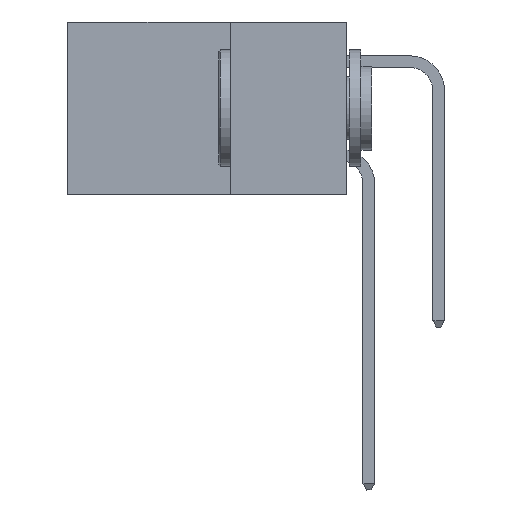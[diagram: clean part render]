
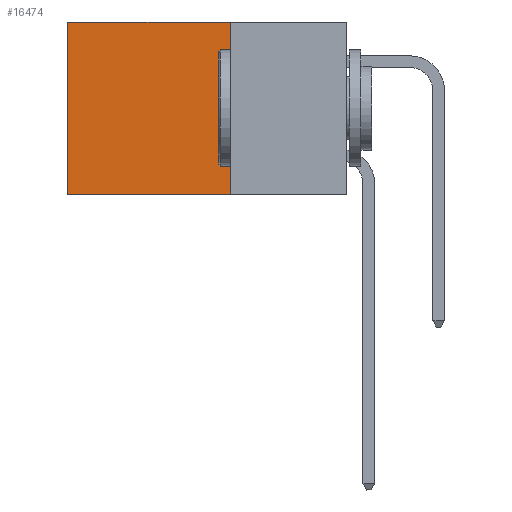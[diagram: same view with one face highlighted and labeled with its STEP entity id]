
A CAD part, left-side view. The second image highlights one B-rep face of the part: STEP entity #16474.
In plain terms, the highlighted planar face has unit normal (-1, 0, 0).
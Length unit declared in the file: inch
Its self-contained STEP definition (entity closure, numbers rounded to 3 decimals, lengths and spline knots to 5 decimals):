
#753 = CARTESIAN_POINT ( 'NONE',  ( 0.2875, 0.6, -0.37 ) ) ;
#780 = DIRECTION ( 'NONE',  ( 0., 1., 0. ) ) ;
#1022 = VECTOR ( 'NONE', #18309, 39.37008 ) ;
#2549 = VERTEX_POINT ( 'NONE', #14756 ) ;
#3037 = DIRECTION ( 'NONE',  ( 1., 0., 0. ) ) ;
#3042 = LINE ( 'NONE', #18124, #1022 ) ;
#4405 = VERTEX_POINT ( 'NONE', #14716 ) ;
#5869 = EDGE_LOOP ( 'NONE', ( #13793, #23216, #25830, #21273 ) ) ;
#6701 = LINE ( 'NONE', #13912, #15279 ) ;
#7751 = VECTOR ( 'NONE', #23376, 39.37008 ) ;
#7761 = CARTESIAN_POINT ( 'NONE',  ( 0.2875, 0.6, 0. ) ) ;
#11403 = DIRECTION ( 'NONE',  ( 0., 0., -1. ) ) ;
#11874 = CARTESIAN_POINT ( 'NONE',  ( 0.2875, 0.25, -0.37 ) ) ;
#12349 = VERTEX_POINT ( 'NONE', #753 ) ;
#12477 = CARTESIAN_POINT ( 'NONE',  ( 0.2875, 0.25, 0. ) ) ;
#13793 = ORIENTED_EDGE ( 'NONE', *, *, #18952, .T. ) ;
#13801 = VERTEX_POINT ( 'NONE', #11874 ) ;
#13912 = CARTESIAN_POINT ( 'NONE',  ( 0.2875, 0.25, -0.37 ) ) ;
#14716 = CARTESIAN_POINT ( 'NONE',  ( 0.2875, 0.6, 0. ) ) ;
#14756 = CARTESIAN_POINT ( 'NONE',  ( 0.2875, 0.25, 0. ) ) ;
#14866 = DIRECTION ( 'NONE',  ( 0., 1., 0. ) ) ;
#15279 = VECTOR ( 'NONE', #780, 39.37008 ) ;
#16161 = FACE_OUTER_BOUND ( 'NONE', #5869, .T. ) ;
#16474 = ADVANCED_FACE ( 'NONE', ( #16161 ), #22448, .F. ) ;
#18124 = CARTESIAN_POINT ( 'NONE',  ( 0.2875, 0.25, 0. ) ) ;
#18309 = DIRECTION ( 'NONE',  ( 0., 0., -1. ) ) ;
#18375 = EDGE_CURVE ( 'NONE', #2549, #13801, #3042, .T. ) ;
#18629 = AXIS2_PLACEMENT_3D ( 'NONE', #26707, #3037, #11403 ) ;
#18952 = EDGE_CURVE ( 'NONE', #4405, #12349, #27146, .T. ) ;
#21273 = ORIENTED_EDGE ( 'NONE', *, *, #23801, .T. ) ;
#22448 = PLANE ( 'NONE',  #18629 ) ;
#23216 = ORIENTED_EDGE ( 'NONE', *, *, #26122, .F. ) ;
#23376 = DIRECTION ( 'NONE',  ( 0., 0., -1. ) ) ;
#23801 = EDGE_CURVE ( 'NONE', #2549, #4405, #26240, .T. ) ;
#24566 = VECTOR ( 'NONE', #14866, 39.37008 ) ;
#25830 = ORIENTED_EDGE ( 'NONE', *, *, #18375, .F. ) ;
#26122 = EDGE_CURVE ( 'NONE', #13801, #12349, #6701, .T. ) ;
#26240 = LINE ( 'NONE', #12477, #24566 ) ;
#26707 = CARTESIAN_POINT ( 'NONE',  ( 0.2875, 0.25, 0. ) ) ;
#27146 = LINE ( 'NONE', #7761, #7751 ) ;
